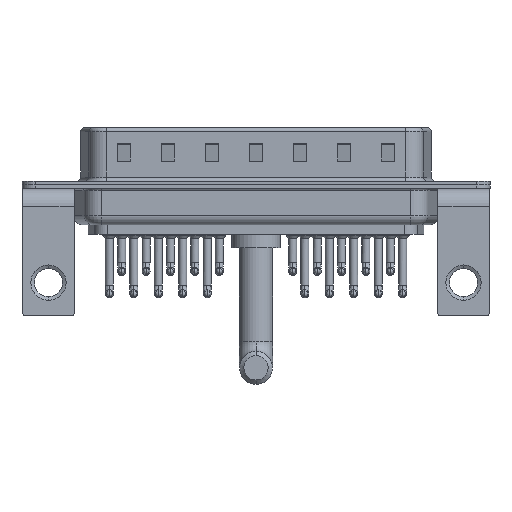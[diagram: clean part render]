
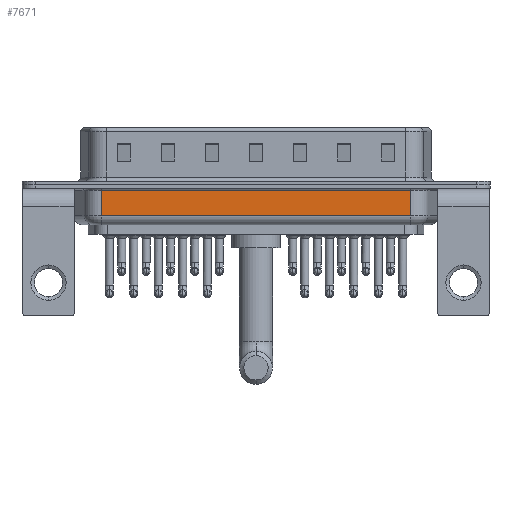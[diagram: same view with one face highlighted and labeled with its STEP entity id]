
A CAD part, front view. The second image highlights one B-rep face of the part: STEP entity #7671.
In plain terms, the highlighted planar face has unit normal (0, -1, 0).
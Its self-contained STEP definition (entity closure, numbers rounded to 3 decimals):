
#400 = CARTESIAN_POINT ( 'NONE',  ( 6.006, -5.35, -4.5 ) ) ;
#1865 = EDGE_CURVE ( 'NONE', #5955, #17233, #14026, .T. ) ;
#1872 = ORIENTED_EDGE ( 'NONE', *, *, #1865, .T. ) ;
#2356 = DIRECTION ( 'NONE',  ( -1., 0., 0. ) ) ;
#2455 = VECTOR ( 'NONE', #9459, 1000. ) ;
#2782 = DIRECTION ( 'NONE',  ( 0., 0., 1. ) ) ;
#5955 = VERTEX_POINT ( 'NONE', #10081 ) ;
#6483 = PLANE ( 'NONE',  #16239 ) ;
#7301 = LINE ( 'NONE', #11347, #2455 ) ;
#7382 = EDGE_CURVE ( 'NONE', #5955, #24156, #7301, .T. ) ;
#7671 = ADVANCED_FACE ( 'NONE', ( #12543 ), #6483, .F. ) ;
#8418 = LINE ( 'NONE', #20814, #22894 ) ;
#9003 = EDGE_LOOP ( 'NONE', ( #20670, #1872, #14161, #21154 ) ) ;
#9459 = DIRECTION ( 'NONE',  ( 0., 0., 1. ) ) ;
#9465 = VERTEX_POINT ( 'NONE', #26127 ) ;
#9836 = CARTESIAN_POINT ( 'NONE',  ( 6.006, -5.35, -3.5 ) ) ;
#10081 = CARTESIAN_POINT ( 'NONE',  ( 6.006, -5.35, -3.5 ) ) ;
#10395 = DIRECTION ( 'NONE',  ( 0., 0., 1. ) ) ;
#11211 = EDGE_CURVE ( 'NONE', #17233, #9465, #17461, .T. ) ;
#11347 = CARTESIAN_POINT ( 'NONE',  ( 6.006, -5.35, -4.5 ) ) ;
#12543 = FACE_OUTER_BOUND ( 'NONE', #9003, .T. ) ;
#12778 = CARTESIAN_POINT ( 'NONE',  ( 41.044, -5.35, -3.5 ) ) ;
#14026 = LINE ( 'NONE', #9836, #26414 ) ;
#14161 = ORIENTED_EDGE ( 'NONE', *, *, #11211, .T. ) ;
#14660 = CARTESIAN_POINT ( 'NONE',  ( 6.006, -5.35, -0.65 ) ) ;
#16239 = AXIS2_PLACEMENT_3D ( 'NONE', #400, #16458, #10395 ) ;
#16458 = DIRECTION ( 'NONE',  ( 0., 1., 0. ) ) ;
#17233 = VERTEX_POINT ( 'NONE', #12778 ) ;
#17461 = LINE ( 'NONE', #21236, #22337 ) ;
#20670 = ORIENTED_EDGE ( 'NONE', *, *, #7382, .F. ) ;
#20814 = CARTESIAN_POINT ( 'NONE',  ( 6.006, -5.35, -0.65 ) ) ;
#21154 = ORIENTED_EDGE ( 'NONE', *, *, #22767, .T. ) ;
#21236 = CARTESIAN_POINT ( 'NONE',  ( 41.044, -5.35, -4.5 ) ) ;
#22337 = VECTOR ( 'NONE', #2782, 1000. ) ;
#22767 = EDGE_CURVE ( 'NONE', #9465, #24156, #8418, .T. ) ;
#22894 = VECTOR ( 'NONE', #2356, 1000. ) ;
#24108 = DIRECTION ( 'NONE',  ( 1., 0., 0. ) ) ;
#24156 = VERTEX_POINT ( 'NONE', #14660 ) ;
#26127 = CARTESIAN_POINT ( 'NONE',  ( 41.044, -5.35, -0.65 ) ) ;
#26414 = VECTOR ( 'NONE', #24108, 1000. ) ;
